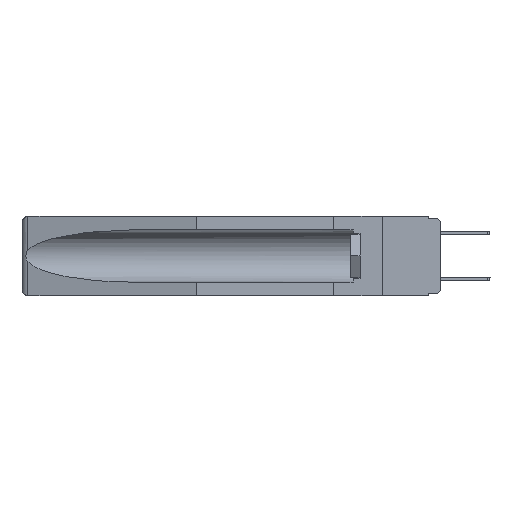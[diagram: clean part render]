
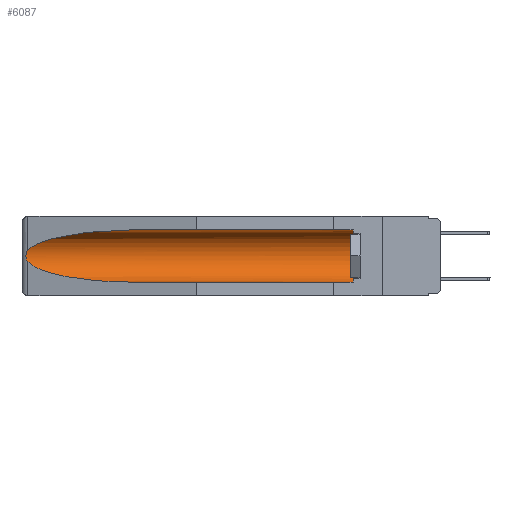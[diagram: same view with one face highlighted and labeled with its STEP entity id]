
A CAD part, left-side view. The second image highlights one B-rep face of the part: STEP entity #6087.
In plain terms, the highlighted cylindrical face has radius 2.857 mm (diameter 5.715 mm), a partial arc.
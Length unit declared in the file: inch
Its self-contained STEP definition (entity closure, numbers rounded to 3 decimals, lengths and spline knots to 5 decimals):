
#690 = CARTESIAN_POINT ( 'NONE',  ( 0.26537, 1.52718, -0.19328 ) ) ;
#1082 = VERTEX_POINT ( 'NONE', #690 ) ;
#1096 = CARTESIAN_POINT ( 'NONE',  ( 0.21114, 1.30732, -0.059 ) ) ;
#1637 = VERTEX_POINT ( 'NONE', #8763 ) ;
#2094 = CARTESIAN_POINT ( 'NONE',  ( 0.26537, 1.52718, -0.14972 ) ) ;
#2830 = DIRECTION ( 'NONE',  ( 0., 1., 0. ) ) ;
#2870 = DIRECTION ( 'NONE',  ( 0., 1., 0. ) ) ;
#3312 = CARTESIAN_POINT ( 'NONE',  ( 0.26654, 1.53092, -0.15636 ) ) ;
#3377 = DIRECTION ( 'NONE',  ( 0., -1., 0. ) ) ;
#3423 = CARTESIAN_POINT ( 'NONE',  ( 0.26655, 1.53094, -0.18657 ) ) ;
#3452 = LINE ( 'NONE', #7997, #13997 ) ;
#3565 = ORIENTED_EDGE ( 'NONE', *, *, #16088, .T. ) ;
#3928 = EDGE_LOOP ( 'NONE', ( #6364, #3565, #12917, #8330, #4326, #12676 ) ) ;
#4275 = VERTEX_POINT ( 'NONE', #11718 ) ;
#4326 = ORIENTED_EDGE ( 'NONE', *, *, #8518, .T. ) ;
#5126 = CARTESIAN_POINT ( 'NONE',  ( 0.155, 1.07973, -0.059 ) ) ;
#5311 = VECTOR ( 'NONE', #14512, 39.37008 ) ;
#5900 =( BOUNDED_CURVE ( )  B_SPLINE_CURVE ( 3, ( #5126, #1096, #6277, #10167 ),
 .UNSPECIFIED., .F., .F. ) 
 B_SPLINE_CURVE_WITH_KNOTS ( ( 4, 4 ),
 ( 4.71239, 6.08839 ),
 .UNSPECIFIED. ) 
 CURVE ( )  GEOMETRIC_REPRESENTATION_ITEM ( )  RATIONAL_B_SPLINE_CURVE ( ( 1., 0.848, 0.848, 1. ) ) 
 REPRESENTATION_ITEM ( '' )  );
#5909 = CARTESIAN_POINT ( 'NONE',  ( 0.2675, 1.53308, -0.16763 ) ) ;
#6033 = EDGE_CURVE ( 'NONE', #1637, #15183, #14044, .T. ) ;
#6087 = ADVANCED_FACE ( 'NONE', ( #8347 ), #8752, .F. ) ;
#6277 = CARTESIAN_POINT ( 'NONE',  ( 0.25451, 1.48313, -0.09465 ) ) ;
#6364 = ORIENTED_EDGE ( 'NONE', *, *, #10864, .T. ) ;
#6850 = DIRECTION ( 'NONE',  ( 0., 0., 1. ) ) ;
#7037 = CARTESIAN_POINT ( 'NONE',  ( 0.155, 1.07973, -0.059 ) ) ;
#7093 = CARTESIAN_POINT ( 'NONE',  ( 0.155, 0.126, -0.284 ) ) ;
#7112 = CARTESIAN_POINT ( 'NONE',  ( 0.2673, 1.5327, -0.16383 ) ) ;
#7997 = CARTESIAN_POINT ( 'NONE',  ( 0.155, -0.30754, -0.284 ) ) ;
#8033 = AXIS2_PLACEMENT_3D ( 'NONE', #9715, #3377, #13756 ) ;
#8330 = ORIENTED_EDGE ( 'NONE', *, *, #15103, .F. ) ;
#8347 = FACE_OUTER_BOUND ( 'NONE', #3928, .T. ) ;
#8457 = CARTESIAN_POINT ( 'NONE',  ( 0.26597, 1.52961, -0.15275 ) ) ;
#8509 = CARTESIAN_POINT ( 'NONE',  ( 0.155, 1.07973, -0.284 ) ) ;
#8518 = EDGE_CURVE ( 'NONE', #16664, #1637, #13181, .T. ) ;
#8752 = CYLINDRICAL_SURFACE ( 'NONE', #16484, 0.1125 ) ;
#8763 = CARTESIAN_POINT ( 'NONE',  ( 0.155, 0.126, -0.059 ) ) ;
#9316 = CARTESIAN_POINT ( 'NONE',  ( 0.155, -0.30754, -0.059 ) ) ;
#9715 = CARTESIAN_POINT ( 'NONE',  ( 0.155, 0.126, -0.1715 ) ) ;
#9824 = CARTESIAN_POINT ( 'NONE',  ( 0.21114, 1.30732, -0.284 ) ) ;
#10012 = CARTESIAN_POINT ( 'NONE',  ( 0.26537, 1.52718, -0.14972 ) ) ;
#10167 = CARTESIAN_POINT ( 'NONE',  ( 0.26537, 1.52718, -0.14972 ) ) ;
#10632 = CARTESIAN_POINT ( 'NONE',  ( 0.155, -0.30754, -0.1715 ) ) ;
#10864 = EDGE_CURVE ( 'NONE', #15183, #13703, #5900, .T. ) ;
#11012 = CARTESIAN_POINT ( 'NONE',  ( 0.25451, 1.48313, -0.24835 ) ) ;
#11057 = CARTESIAN_POINT ( 'NONE',  ( 0.26537, 1.52718, -0.19328 ) ) ;
#11718 = CARTESIAN_POINT ( 'NONE',  ( 0.155, 1.07973, -0.284 ) ) ;
#12442 =( BOUNDED_CURVE ( )  B_SPLINE_CURVE ( 3, ( #11057, #11012, #9824, #8509 ),
 .UNSPECIFIED., .F., .T. ) 
 B_SPLINE_CURVE_WITH_KNOTS ( ( 4, 4 ),
 ( 0.1948, 1.5708 ),
 .UNSPECIFIED. ) 
 CURVE ( )  GEOMETRIC_REPRESENTATION_ITEM ( )  RATIONAL_B_SPLINE_CURVE ( ( 1., 0.848, 0.848, 1. ) ) 
 REPRESENTATION_ITEM ( '' )  );
#12676 = ORIENTED_EDGE ( 'NONE', *, *, #6033, .T. ) ;
#12917 = ORIENTED_EDGE ( 'NONE', *, *, #16113, .T. ) ;
#13181 = CIRCLE ( 'NONE', #8033, 0.1125 ) ;
#13703 = VERTEX_POINT ( 'NONE', #10012 ) ;
#13756 = DIRECTION ( 'NONE',  ( 0., 0., 1. ) ) ;
#13860 = CARTESIAN_POINT ( 'NONE',  ( 0.2673, 1.53269, -0.17917 ) ) ;
#13997 = VECTOR ( 'NONE', #2830, 39.37008 ) ;
#14044 = LINE ( 'NONE', #9316, #5311 ) ;
#14512 = DIRECTION ( 'NONE',  ( 0., 1., 0. ) ) ;
#14985 = CARTESIAN_POINT ( 'NONE',  ( 0.2675, 1.53308, -0.17534 ) ) ;
#15103 = EDGE_CURVE ( 'NONE', #16664, #4275, #3452, .T. ) ;
#15183 = VERTEX_POINT ( 'NONE', #7037 ) ;
#15482 = B_SPLINE_CURVE_WITH_KNOTS ( 'NONE', 3,
 ( #2094, #8457, #3312, #7112, #5909, #14985, #13860, #3423, #16283, #16181 ),
 .UNSPECIFIED., .F., .F.,
 ( 4, 2, 2, 2, 4 ),
 ( 0., 0.00029, 0.00058, 0.00087, 0.00117 ),
 .UNSPECIFIED. ) ;
#16088 = EDGE_CURVE ( 'NONE', #13703, #1082, #15482, .T. ) ;
#16113 = EDGE_CURVE ( 'NONE', #1082, #4275, #12442, .T. ) ;
#16181 = CARTESIAN_POINT ( 'NONE',  ( 0.26537, 1.52718, -0.19328 ) ) ;
#16283 = CARTESIAN_POINT ( 'NONE',  ( 0.26597, 1.5296, -0.19026 ) ) ;
#16484 = AXIS2_PLACEMENT_3D ( 'NONE', #10632, #2870, #6850 ) ;
#16664 = VERTEX_POINT ( 'NONE', #7093 ) ;
